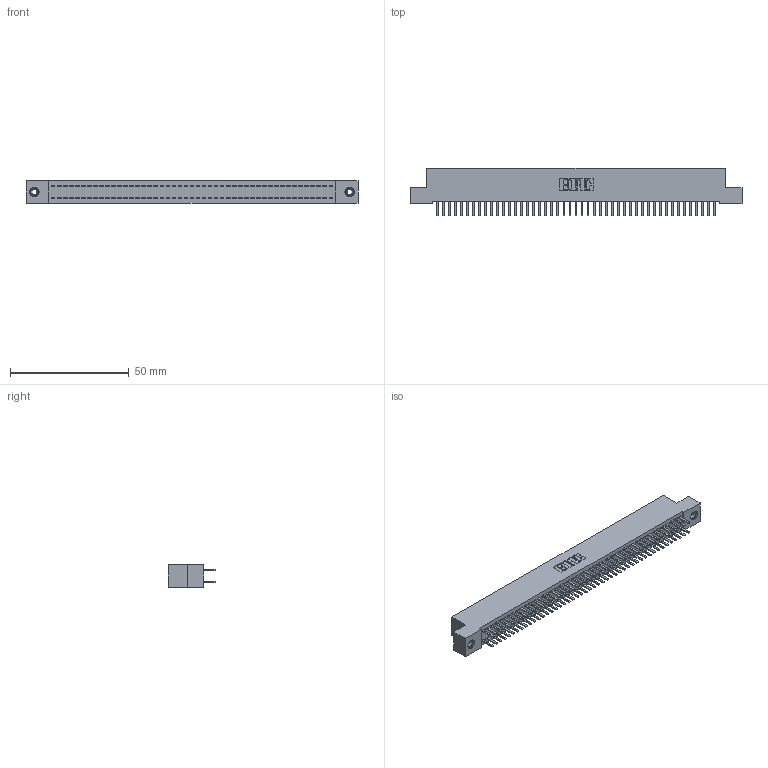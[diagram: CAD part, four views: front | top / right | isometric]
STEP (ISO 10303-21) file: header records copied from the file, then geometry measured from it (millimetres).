
FILE_DESCRIPTION (( 'STEP AP203' ), '1' );
FILE_NAME ('392-094-520-208.STEP', '2019-10-09T19:12:36', ( '' ), ( '' ), 'SwSTEP 2.0', 'SolidWorks 2016', '' );
FILE_SCHEMA (( 'CONFIG_CONTROL_DESIGN' ));
Length unit declared in the file: inch
Products named in the file (4): 342 Part_TI; 345-292-001_345-293-120; 345-250-001_345-250-003-102; 392-094-520-208
Assembly tree (97 placements, depth 2):
  392-094-520-208
    342 Part_TI
    345-292-001_345-293-120  x94
    345-250-001_345-250-003-102  x2
Bounding box: 139.7 x 20.02 x 9.4 mm (x, y, z)
Volume: 12528.7 mm3; surface area: 20429.6 mm2
Topology: 97 solids, 97 shells, 5434 faces, 15757 edges, 10246 vertices
Faces by surface type: plane 3670, cylinder 1748, cone 12, torus 4
Entity records: 30758 total; most frequent: CARTESIAN_POINT 5085, ORIENTED_EDGE 5002, DIRECTION 4355, EDGE_CURVE 2501, VECTOR 2349, LINE 2349, VERTEX_POINT 1660, AXIS2_PLACEMENT_3D 1003
